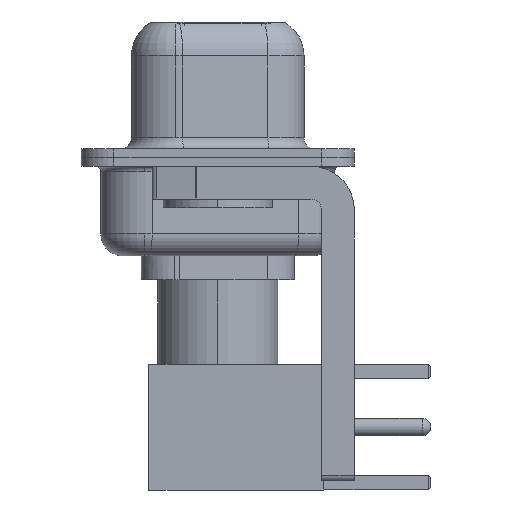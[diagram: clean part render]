
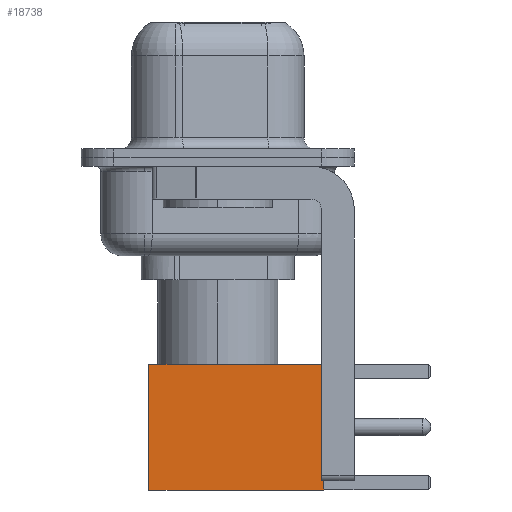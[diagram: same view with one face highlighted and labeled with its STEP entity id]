
A CAD part, left-side view. The second image highlights one B-rep face of the part: STEP entity #18738.
In plain terms, the highlighted face is planar.
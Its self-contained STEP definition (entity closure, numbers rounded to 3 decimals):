
#649 = LINE ( 'NONE', #13983, #2513 ) ;
#676 = DIRECTION ( 'NONE',  ( 0., 0., 1. ) ) ;
#1793 = CARTESIAN_POINT ( 'NONE',  ( -2.875, 2.875, 8. ) ) ;
#1819 = CARTESIAN_POINT ( 'NONE',  ( 0., 2.875, 8. ) ) ;
#2277 = DIRECTION ( 'NONE',  ( 0., 0., -1. ) ) ;
#2454 = CARTESIAN_POINT ( 'NONE',  ( 2.875, 2.875, 8. ) ) ;
#2513 = VECTOR ( 'NONE', #12706, 1000. ) ;
#3050 = ORIENTED_EDGE ( 'NONE', *, *, #16309, .F. ) ;
#3181 = CARTESIAN_POINT ( 'NONE',  ( 2.875, 2.875, 0. ) ) ;
#3442 = LINE ( 'NONE', #6746, #5645 ) ;
#5581 = ORIENTED_EDGE ( 'NONE', *, *, #6626, .F. ) ;
#5645 = VECTOR ( 'NONE', #2277, 1000. ) ;
#6162 = DIRECTION ( 'NONE',  ( -1., 0., 0. ) ) ;
#6202 = VERTEX_POINT ( 'NONE', #12917 ) ;
#6359 = LINE ( 'NONE', #10358, #8053 ) ;
#6492 = FACE_OUTER_BOUND ( 'NONE', #8324, .T. ) ;
#6626 = EDGE_CURVE ( 'NONE', #14666, #6202, #3442, .T. ) ;
#6690 = CARTESIAN_POINT ( 'NONE',  ( 2.875, 2.875, 0. ) ) ;
#6746 = CARTESIAN_POINT ( 'NONE',  ( -2.875, 2.875, 0. ) ) ;
#7062 = ORIENTED_EDGE ( 'NONE', *, *, #12461, .T. ) ;
#7630 = AXIS2_PLACEMENT_3D ( 'NONE', #6690, #18485, #676 ) ;
#8053 = VECTOR ( 'NONE', #6162, 1000. ) ;
#8118 = VERTEX_POINT ( 'NONE', #3181 ) ;
#8324 = EDGE_LOOP ( 'NONE', ( #7062, #13998, #5581, #3050 ) ) ;
#10081 = EDGE_CURVE ( 'NONE', #8118, #6202, #6359, .T. ) ;
#10358 = CARTESIAN_POINT ( 'NONE',  ( 0., 2.875, 0. ) ) ;
#12461 = EDGE_CURVE ( 'NONE', #19224, #8118, #649, .T. ) ;
#12706 = DIRECTION ( 'NONE',  ( 0., 0., -1. ) ) ;
#12917 = CARTESIAN_POINT ( 'NONE',  ( -2.875, 2.875, 0. ) ) ;
#13710 = PLANE ( 'NONE',  #7630 ) ;
#13983 = CARTESIAN_POINT ( 'NONE',  ( 2.875, 2.875, 0. ) ) ;
#13998 = ORIENTED_EDGE ( 'NONE', *, *, #10081, .T. ) ;
#14666 = VERTEX_POINT ( 'NONE', #1793 ) ;
#16309 = EDGE_CURVE ( 'NONE', #19224, #14666, #16723, .T. ) ;
#16723 = LINE ( 'NONE', #1819, #16943 ) ;
#16943 = VECTOR ( 'NONE', #18377, 1000. ) ;
#18377 = DIRECTION ( 'NONE',  ( -1., 0., 0. ) ) ;
#18485 = DIRECTION ( 'NONE',  ( 0., 1., 0. ) ) ;
#18738 = ADVANCED_FACE ( 'NONE', ( #6492 ), #13710, .T. ) ;
#19224 = VERTEX_POINT ( 'NONE', #2454 ) ;
